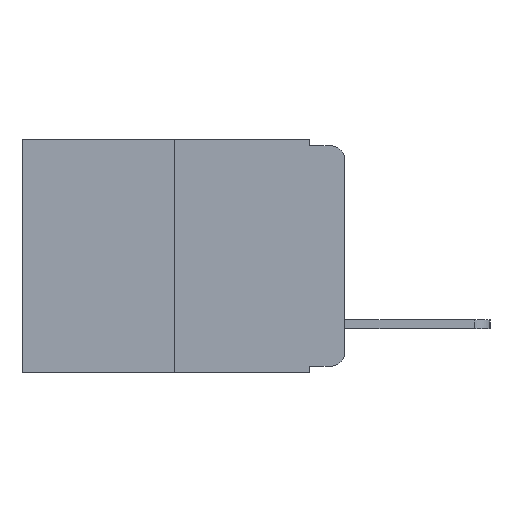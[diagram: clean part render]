
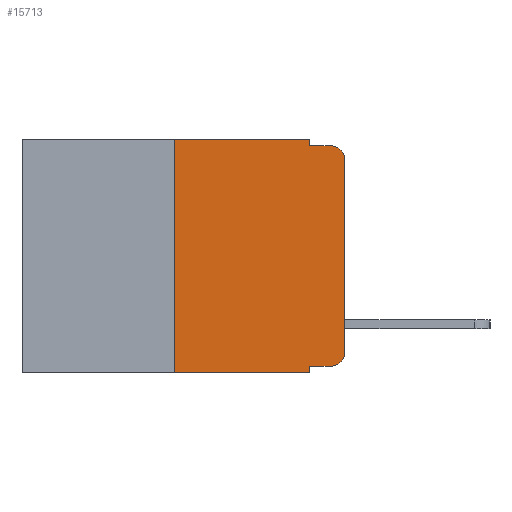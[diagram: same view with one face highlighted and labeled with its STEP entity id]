
A CAD part, left-side view. The second image highlights one B-rep face of the part: STEP entity #15713.
In plain terms, the highlighted planar face has unit normal (-1, 0, 0).
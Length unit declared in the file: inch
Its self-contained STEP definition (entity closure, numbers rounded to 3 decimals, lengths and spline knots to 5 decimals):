
#140 = DIRECTION ( 'NONE',  ( 1., 0., 0. ) ) ;
#465 = VECTOR ( 'NONE', #18753, 39.37008 ) ;
#799 = EDGE_CURVE ( 'NONE', #13174, #24185, #6618, .T. ) ;
#1222 = VERTEX_POINT ( 'NONE', #21497 ) ;
#1282 = VECTOR ( 'NONE', #13758, 39.37008 ) ;
#1440 = AXIS2_PLACEMENT_3D ( 'NONE', #14151, #140, #14237 ) ;
#1951 = LINE ( 'NONE', #11717, #1282 ) ;
#2214 = EDGE_CURVE ( 'NONE', #21409, #1222, #5899, .T. ) ;
#2276 = ORIENTED_EDGE ( 'NONE', *, *, #7805, .F. ) ;
#2303 = ORIENTED_EDGE ( 'NONE', *, *, #2214, .F. ) ;
#2339 = VECTOR ( 'NONE', #23845, 39.37008 ) ;
#3061 = VERTEX_POINT ( 'NONE', #25333 ) ;
#3378 = CARTESIAN_POINT ( 'NONE',  ( 0., 0.02, -0.01 ) ) ;
#3647 = ORIENTED_EDGE ( 'NONE', *, *, #25413, .F. ) ;
#3934 = EDGE_CURVE ( 'NONE', #13174, #4894, #12216, .T. ) ;
#4894 = VERTEX_POINT ( 'NONE', #15654 ) ;
#4915 = EDGE_CURVE ( 'NONE', #1222, #21699, #7517, .T. ) ;
#5549 = AXIS2_PLACEMENT_3D ( 'NONE', #23919, #12005, #25886 ) ;
#5847 = EDGE_LOOP ( 'NONE', ( #17176, #16862, #13305, #2303, #2276, #13243, #24225, #3647, #7772, #22514 ) ) ;
#5861 = CARTESIAN_POINT ( 'NONE',  ( 0., 0.051, -0.333 ) ) ;
#5899 = LINE ( 'NONE', #24607, #465 ) ;
#6170 = CARTESIAN_POINT ( 'NONE',  ( 0., 0.25, -0.343 ) ) ;
#6295 = EDGE_CURVE ( 'NONE', #9411, #21699, #16820, .T. ) ;
#6427 = LINE ( 'NONE', #23380, #15765 ) ;
#6485 = CARTESIAN_POINT ( 'NONE',  ( 0., 0.02, -0.333 ) ) ;
#6618 = LINE ( 'NONE', #9864, #20670 ) ;
#7517 = LINE ( 'NONE', #13749, #17518 ) ;
#7615 = EDGE_CURVE ( 'NONE', #3061, #9411, #20801, .T. ) ;
#7772 = ORIENTED_EDGE ( 'NONE', *, *, #24107, .T. ) ;
#7805 = EDGE_CURVE ( 'NONE', #24185, #21409, #6427, .T. ) ;
#7836 = DIRECTION ( 'NONE',  ( -1., 0., 0. ) ) ;
#8065 = VERTEX_POINT ( 'NONE', #6485 ) ;
#9411 = VERTEX_POINT ( 'NONE', #19147 ) ;
#9864 = CARTESIAN_POINT ( 'NONE',  ( 0., 0.25, 0. ) ) ;
#10570 = FACE_OUTER_BOUND ( 'NONE', #5847, .T. ) ;
#10941 = VECTOR ( 'NONE', #22169, 39.37008 ) ;
#11708 = DIRECTION ( 'NONE',  ( 0., -1., 0. ) ) ;
#11717 = CARTESIAN_POINT ( 'NONE',  ( 0., 0.051, 0. ) ) ;
#11894 = DIRECTION ( 'NONE',  ( 0., 0., 1. ) ) ;
#11934 = CARTESIAN_POINT ( 'NONE',  ( 0., 0.051, -0.333 ) ) ;
#12005 = DIRECTION ( 'NONE',  ( -1., 0., 0. ) ) ;
#12216 = LINE ( 'NONE', #12219, #10941 ) ;
#12219 = CARTESIAN_POINT ( 'NONE',  ( 0., 0.473, -0.343 ) ) ;
#12235 = PLANE ( 'NONE',  #1440 ) ;
#12410 = CARTESIAN_POINT ( 'NONE',  ( 0., 0.051, 0. ) ) ;
#13174 = VERTEX_POINT ( 'NONE', #6170 ) ;
#13243 = ORIENTED_EDGE ( 'NONE', *, *, #799, .F. ) ;
#13305 = ORIENTED_EDGE ( 'NONE', *, *, #4915, .F. ) ;
#13692 = CIRCLE ( 'NONE', #14705, 0.02 ) ;
#13749 = CARTESIAN_POINT ( 'NONE',  ( 0., 0.051, -0.01 ) ) ;
#13758 = DIRECTION ( 'NONE',  ( 0., 0., -1. ) ) ;
#14151 = CARTESIAN_POINT ( 'NONE',  ( 0., 0.473, 0. ) ) ;
#14212 = CARTESIAN_POINT ( 'NONE',  ( 0., 0.25, 0. ) ) ;
#14237 = DIRECTION ( 'NONE',  ( 0., 0., -1. ) ) ;
#14705 = AXIS2_PLACEMENT_3D ( 'NONE', #19808, #7836, #21790 ) ;
#15468 = VECTOR ( 'NONE', #20830, 39.37008 ) ;
#15469 = DIRECTION ( 'NONE',  ( 0., -1., 0. ) ) ;
#15654 = CARTESIAN_POINT ( 'NONE',  ( 0., 0.051, -0.343 ) ) ;
#15713 = ADVANCED_FACE ( 'NONE', ( #10570 ), #12235, .F. ) ;
#15765 = VECTOR ( 'NONE', #15469, 39.37008 ) ;
#16820 = CIRCLE ( 'NONE', #5549, 0.02 ) ;
#16862 = ORIENTED_EDGE ( 'NONE', *, *, #6295, .T. ) ;
#17176 = ORIENTED_EDGE ( 'NONE', *, *, #7615, .T. ) ;
#17395 = VERTEX_POINT ( 'NONE', #5861 ) ;
#17518 = VECTOR ( 'NONE', #11708, 39.37008 ) ;
#18321 = LINE ( 'NONE', #11934, #2339 ) ;
#18753 = DIRECTION ( 'NONE',  ( 0., 0., -1. ) ) ;
#19147 = CARTESIAN_POINT ( 'NONE',  ( 0., 0., -0.03 ) ) ;
#19808 = CARTESIAN_POINT ( 'NONE',  ( 0., 0.02, -0.313 ) ) ;
#20670 = VECTOR ( 'NONE', #11894, 39.37008 ) ;
#20801 = LINE ( 'NONE', #24676, #15468 ) ;
#20830 = DIRECTION ( 'NONE',  ( 0., 0., 1. ) ) ;
#21409 = VERTEX_POINT ( 'NONE', #12410 ) ;
#21497 = CARTESIAN_POINT ( 'NONE',  ( 0., 0.051, -0.01 ) ) ;
#21699 = VERTEX_POINT ( 'NONE', #3378 ) ;
#21790 = DIRECTION ( 'NONE',  ( 0., 0., -1. ) ) ;
#22169 = DIRECTION ( 'NONE',  ( 0., -1., 0. ) ) ;
#22514 = ORIENTED_EDGE ( 'NONE', *, *, #22802, .T. ) ;
#22802 = EDGE_CURVE ( 'NONE', #8065, #3061, #13692, .T. ) ;
#23380 = CARTESIAN_POINT ( 'NONE',  ( 0., 0.473, 0. ) ) ;
#23845 = DIRECTION ( 'NONE',  ( 0., -1., 0. ) ) ;
#23919 = CARTESIAN_POINT ( 'NONE',  ( 0., 0.02, -0.03 ) ) ;
#24107 = EDGE_CURVE ( 'NONE', #17395, #8065, #18321, .T. ) ;
#24185 = VERTEX_POINT ( 'NONE', #14212 ) ;
#24225 = ORIENTED_EDGE ( 'NONE', *, *, #3934, .T. ) ;
#24607 = CARTESIAN_POINT ( 'NONE',  ( 0., 0.051, 0. ) ) ;
#24676 = CARTESIAN_POINT ( 'NONE',  ( 0., 0., 0. ) ) ;
#25333 = CARTESIAN_POINT ( 'NONE',  ( 0., 0., -0.313 ) ) ;
#25413 = EDGE_CURVE ( 'NONE', #17395, #4894, #1951, .T. ) ;
#25886 = DIRECTION ( 'NONE',  ( 0., 0., -1. ) ) ;
